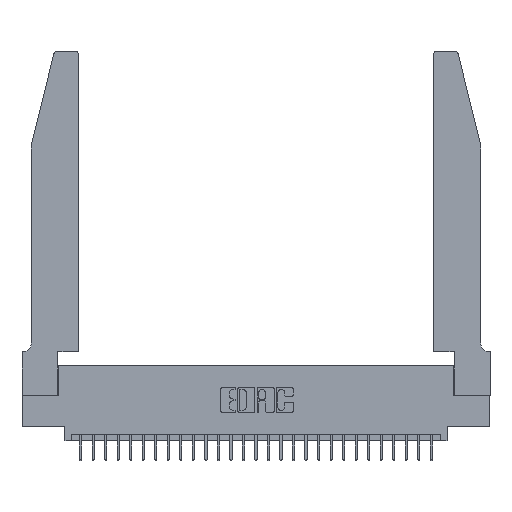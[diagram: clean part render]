
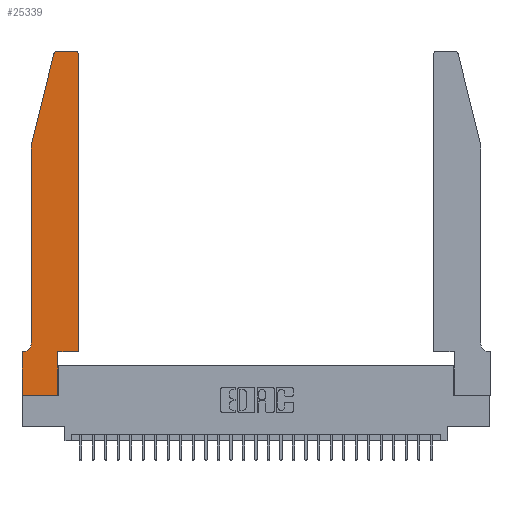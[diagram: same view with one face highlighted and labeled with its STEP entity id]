
A CAD part, top view. The second image highlights one B-rep face of the part: STEP entity #25339.
In plain terms, the highlighted planar face has unit normal (0, 0, 1).
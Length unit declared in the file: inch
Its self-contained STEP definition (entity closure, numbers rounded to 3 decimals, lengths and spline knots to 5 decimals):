
#56 = VECTOR ( 'NONE', #2867, 39.37008 ) ;
#263 = CARTESIAN_POINT ( 'NONE',  ( 0.2865, 0., 0.37 ) ) ;
#686 = VERTEX_POINT ( 'NONE', #20263 ) ;
#793 = ORIENTED_EDGE ( 'NONE', *, *, #14101, .T. ) ;
#1210 = CARTESIAN_POINT ( 'NONE',  ( 0., 0., 0.37 ) ) ;
#1335 = VERTEX_POINT ( 'NONE', #1210 ) ;
#1716 = CIRCLE ( 'NONE', #7692, 0.03 ) ;
#2041 = EDGE_CURVE ( 'NONE', #22668, #19924, #21652, .T. ) ;
#2545 = DIRECTION ( 'NONE',  ( 0., 0., 1. ) ) ;
#2867 = DIRECTION ( 'NONE',  ( -1., 0., 0. ) ) ;
#2942 = LINE ( 'NONE', #20030, #19736 ) ;
#2959 = CARTESIAN_POINT ( 'NONE',  ( 0.0755, 2., 0.37 ) ) ;
#3954 = CARTESIAN_POINT ( 'NONE',  ( 0.2865, 0.35, 0.37 ) ) ;
#4279 = LINE ( 'NONE', #5321, #21764 ) ;
#4393 = ORIENTED_EDGE ( 'NONE', *, *, #27930, .T. ) ;
#5055 = CIRCLE ( 'NONE', #11672, 0.07 ) ;
#5318 = VECTOR ( 'NONE', #5756, 39.37008 ) ;
#5321 = CARTESIAN_POINT ( 'NONE',  ( 0., 0., 0.37 ) ) ;
#5756 = DIRECTION ( 'NONE',  ( 0., -1., 0. ) ) ;
#5960 = LINE ( 'NONE', #8133, #12085 ) ;
#6488 = DIRECTION ( 'NONE',  ( 0., 0., 1. ) ) ;
#6630 = ORIENTED_EDGE ( 'NONE', *, *, #2041, .T. ) ;
#6951 = DIRECTION ( 'NONE',  ( 0., 0., -1. ) ) ;
#7158 = LINE ( 'NONE', #10997, #12519 ) ;
#7413 = LINE ( 'NONE', #2959, #13486 ) ;
#7692 = AXIS2_PLACEMENT_3D ( 'NONE', #20110, #6488, #22375 ) ;
#8030 = ORIENTED_EDGE ( 'NONE', *, *, #25561, .T. ) ;
#8062 = ORIENTED_EDGE ( 'NONE', *, *, #23117, .T. ) ;
#8091 = EDGE_CURVE ( 'NONE', #18199, #21626, #1716, .T. ) ;
#8125 = CARTESIAN_POINT ( 'NONE',  ( 0.0755, 2., 0.37 ) ) ;
#8133 = CARTESIAN_POINT ( 'NONE',  ( 0.2605, 2.75, 0.37 ) ) ;
#9741 = EDGE_CURVE ( 'NONE', #19924, #18199, #5960, .T. ) ;
#9757 = DIRECTION ( 'NONE',  ( 0., 0., 1. ) ) ;
#9843 = DIRECTION ( 'NONE',  ( -0.239, -0.971, 0. ) ) ;
#10104 = CARTESIAN_POINT ( 'NONE',  ( 0.2865, 0.35, 0.37 ) ) ;
#10880 = EDGE_CURVE ( 'NONE', #21626, #18473, #7413, .T. ) ;
#10889 = LINE ( 'NONE', #20423, #22207 ) ;
#10997 = CARTESIAN_POINT ( 'NONE',  ( 0.4505, 0.35, 0.37 ) ) ;
#11672 = AXIS2_PLACEMENT_3D ( 'NONE', #20546, #6951, #22808 ) ;
#12013 = VERTEX_POINT ( 'NONE', #263 ) ;
#12085 = VECTOR ( 'NONE', #14890, 39.37008 ) ;
#12275 = DIRECTION ( 'NONE',  ( 1., 0., 0. ) ) ;
#12342 = CARTESIAN_POINT ( 'NONE',  ( 0.4205, 2.75, 0.37 ) ) ;
#12398 = DIRECTION ( 'NONE',  ( 0., 1., 0. ) ) ;
#12519 = VECTOR ( 'NONE', #15678, 39.37008 ) ;
#13486 = VECTOR ( 'NONE', #9843, 39.37008 ) ;
#13553 = CARTESIAN_POINT ( 'NONE',  ( 0.4505, 0.35, 0.37 ) ) ;
#14101 = EDGE_CURVE ( 'NONE', #1335, #12013, #4279, .T. ) ;
#14282 = AXIS2_PLACEMENT_3D ( 'NONE', #25228, #2545, #18537 ) ;
#14335 = CARTESIAN_POINT ( 'NONE',  ( 0.0755, 0.35, 0.37 ) ) ;
#14480 = ORIENTED_EDGE ( 'NONE', *, *, #28869, .T. ) ;
#14890 = DIRECTION ( 'NONE',  ( -1., 0., 0. ) ) ;
#15678 = DIRECTION ( 'NONE',  ( 0., 1., 0. ) ) ;
#15908 = ORIENTED_EDGE ( 'NONE', *, *, #23211, .T. ) ;
#15921 = CARTESIAN_POINT ( 'NONE',  ( 0.25487, 2.72718, 0.37 ) ) ;
#17988 = ORIENTED_EDGE ( 'NONE', *, *, #22746, .T. ) ;
#18199 = VERTEX_POINT ( 'NONE', #28291 ) ;
#18473 = VERTEX_POINT ( 'NONE', #27301 ) ;
#18537 = DIRECTION ( 'NONE',  ( 1., 0., 0. ) ) ;
#18842 = VERTEX_POINT ( 'NONE', #3954 ) ;
#19015 = ORIENTED_EDGE ( 'NONE', *, *, #8091, .T. ) ;
#19736 = VECTOR ( 'NONE', #24545, 39.37008 ) ;
#19769 = LINE ( 'NONE', #14335, #56 ) ;
#19924 = VERTEX_POINT ( 'NONE', #12342 ) ;
#20030 = CARTESIAN_POINT ( 'NONE',  ( 0., 0., 0.37 ) ) ;
#20110 = CARTESIAN_POINT ( 'NONE',  ( 0.284, 2.72, 0.37 ) ) ;
#20263 = CARTESIAN_POINT ( 'NONE',  ( 0.0755, 0.42, 0.37 ) ) ;
#20423 = CARTESIAN_POINT ( 'NONE',  ( 0.4505, 0.35, 0.37 ) ) ;
#20546 = CARTESIAN_POINT ( 'NONE',  ( 0.0055, 0.42, 0.37 ) ) ;
#20720 = PLANE ( 'NONE',  #14282 ) ;
#21626 = VERTEX_POINT ( 'NONE', #15921 ) ;
#21652 = CIRCLE ( 'NONE', #22407, 0.03 ) ;
#21764 = VECTOR ( 'NONE', #12275, 39.37008 ) ;
#22160 = LINE ( 'NONE', #10104, #23554 ) ;
#22207 = VECTOR ( 'NONE', #22691, 39.37008 ) ;
#22271 = CARTESIAN_POINT ( 'NONE',  ( 0.0055, 0.35, 0.37 ) ) ;
#22375 = DIRECTION ( 'NONE',  ( 1., 0., 0. ) ) ;
#22407 = AXIS2_PLACEMENT_3D ( 'NONE', #23290, #9757, #25546 ) ;
#22527 = VERTEX_POINT ( 'NONE', #13553 ) ;
#22668 = VERTEX_POINT ( 'NONE', #27616 ) ;
#22691 = DIRECTION ( 'NONE',  ( 1., 0., 0. ) ) ;
#22746 = EDGE_CURVE ( 'NONE', #23750, #23783, #19769, .T. ) ;
#22808 = DIRECTION ( 'NONE',  ( -1., 0., 0. ) ) ;
#23117 = EDGE_CURVE ( 'NONE', #23783, #1335, #2942, .T. ) ;
#23211 = EDGE_CURVE ( 'NONE', #18842, #22527, #10889, .T. ) ;
#23290 = CARTESIAN_POINT ( 'NONE',  ( 0.4205, 2.72, 0.37 ) ) ;
#23463 = LINE ( 'NONE', #8125, #5318 ) ;
#23554 = VECTOR ( 'NONE', #12398, 39.37008 ) ;
#23750 = VERTEX_POINT ( 'NONE', #22271 ) ;
#23783 = VERTEX_POINT ( 'NONE', #26864 ) ;
#24545 = DIRECTION ( 'NONE',  ( 0., -1., 0. ) ) ;
#25228 = CARTESIAN_POINT ( 'NONE',  ( 0., 0.35, 0.37 ) ) ;
#25339 = ADVANCED_FACE ( 'NONE', ( #28383 ), #20720, .T. ) ;
#25546 = DIRECTION ( 'NONE',  ( 1., 0., 0. ) ) ;
#25561 = EDGE_CURVE ( 'NONE', #18473, #686, #23463, .T. ) ;
#25732 = EDGE_CURVE ( 'NONE', #22527, #22668, #7158, .T. ) ;
#26864 = CARTESIAN_POINT ( 'NONE',  ( 0., 0.35, 0.37 ) ) ;
#27301 = CARTESIAN_POINT ( 'NONE',  ( 0.0755, 2., 0.37 ) ) ;
#27571 = EDGE_LOOP ( 'NONE', ( #28129, #19015, #27793, #8030, #4393, #17988, #8062, #793, #14480, #15908, #28550, #6630 ) ) ;
#27616 = CARTESIAN_POINT ( 'NONE',  ( 0.4505, 2.72, 0.37 ) ) ;
#27793 = ORIENTED_EDGE ( 'NONE', *, *, #10880, .T. ) ;
#27930 = EDGE_CURVE ( 'NONE', #686, #23750, #5055, .T. ) ;
#28129 = ORIENTED_EDGE ( 'NONE', *, *, #9741, .T. ) ;
#28291 = CARTESIAN_POINT ( 'NONE',  ( 0.284, 2.75, 0.37 ) ) ;
#28383 = FACE_OUTER_BOUND ( 'NONE', #27571, .T. ) ;
#28550 = ORIENTED_EDGE ( 'NONE', *, *, #25732, .T. ) ;
#28869 = EDGE_CURVE ( 'NONE', #12013, #18842, #22160, .T. ) ;
